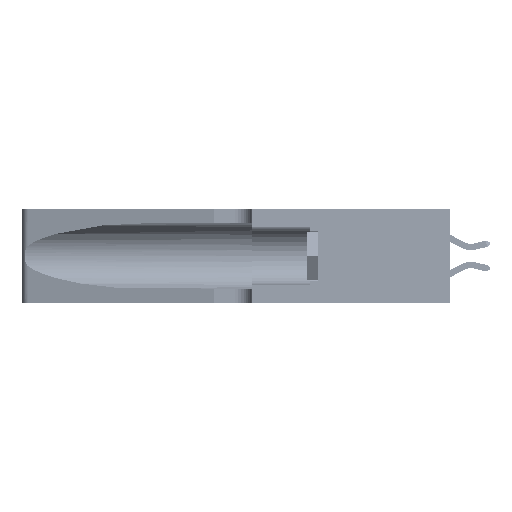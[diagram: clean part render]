
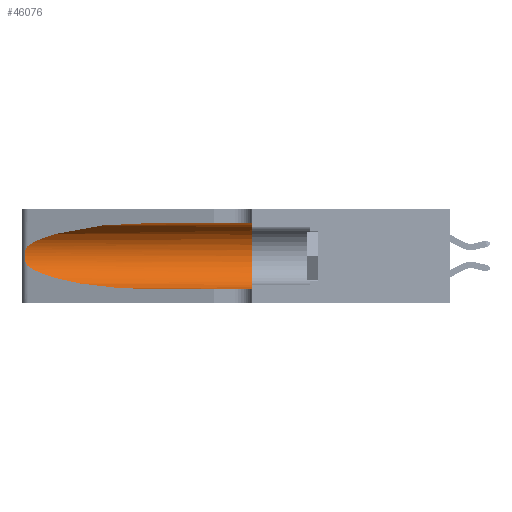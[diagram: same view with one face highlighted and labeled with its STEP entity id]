
A CAD part, left-side view. The second image highlights one B-rep face of the part: STEP entity #46076.
In plain terms, the highlighted cylindrical face has radius 3.308 mm (diameter 6.617 mm), a partial arc.
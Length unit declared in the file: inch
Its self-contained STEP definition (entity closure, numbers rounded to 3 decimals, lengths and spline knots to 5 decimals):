
#816 = DIRECTION ( 'NONE',  ( 0., 0., 1. ) ) ;
#819 = ORIENTED_EDGE ( 'NONE', *, *, #31638, .T. ) ;
#899 = CARTESIAN_POINT ( 'NONE',  ( 0.26075, 1.23896, 0.178 ) ) ;
#1541 = VERTEX_POINT ( 'NONE', #27098 ) ;
#3006 = FACE_OUTER_BOUND ( 'NONE', #21736, .T. ) ;
#5270 = CARTESIAN_POINT ( 'NONE',  ( 0.25856, 1.23593, 0.16098 ) ) ;
#9612 = CARTESIAN_POINT ( 'NONE',  ( 0.25639, 1.23186, 0.15144 ) ) ;
#9750 = AXIS2_PLACEMENT_3D ( 'NONE', #45708, #20847, #29178 ) ;
#10561 = CARTESIAN_POINT ( 'NONE',  ( 0.18966, 0.96281, 0.31525 ) ) ;
#13496 = ORIENTED_EDGE ( 'NONE', *, *, #45112, .T. ) ;
#13919 = CARTESIAN_POINT ( 'NONE',  ( 0.25487, 1.22718, 0.14631 ) ) ;
#15225 = CARTESIAN_POINT ( 'NONE',  ( 0.25487, 1.22718, 0.14631 ) ) ;
#15286 = CARTESIAN_POINT ( 'NONE',  ( 0.1305, 0.72297, 0.31525 ) ) ;
#15536 = ORIENTED_EDGE ( 'NONE', *, *, #39988, .F. ) ;
#18020 = CARTESIAN_POINT ( 'NONE',  ( 0.25639, 1.23184, 0.21858 ) ) ;
#19123 = CARTESIAN_POINT ( 'NONE',  ( 0.1305, 0.72297, 0.31525 ) ) ;
#19491 = CARTESIAN_POINT ( 'NONE',  ( 0.2373, 1.15595, 0.08982 ) ) ;
#20099 =( BOUNDED_CURVE ( )  B_SPLINE_CURVE ( 3, ( #19123, #10561, #39635, #48132 ),
 .UNSPECIFIED., .F., .F. ) 
 B_SPLINE_CURVE_WITH_KNOTS ( ( 4, 4 ),
 ( 1.5708, 2.84003 ),
 .UNSPECIFIED. ) 
 CURVE ( )  GEOMETRIC_REPRESENTATION_ITEM ( )  RATIONAL_B_SPLINE_CURVE ( ( 1., 0.87, 0.87, 1. ) ) 
 REPRESENTATION_ITEM ( '' )  );
#20847 = DIRECTION ( 'NONE',  ( 0., -1., 0. ) ) ;
#20879 = CARTESIAN_POINT ( 'NONE',  ( 0.25487, 1.22718, 0.22369 ) ) ;
#21736 = EDGE_LOOP ( 'NONE', ( #52640, #13496, #819, #24892, #15536, #44374 ) ) ;
#22223 = CARTESIAN_POINT ( 'NONE',  ( 0.25854, 1.2359, 0.20912 ) ) ;
#23657 = CARTESIAN_POINT ( 'NONE',  ( 0.1305, 0.72297, 0.05475 ) ) ;
#24892 = ORIENTED_EDGE ( 'NONE', *, *, #35513, .T. ) ;
#25567 = EDGE_CURVE ( 'NONE', #27614, #38202, #27658, .T. ) ;
#25776 = VERTEX_POINT ( 'NONE', #36055 ) ;
#25979 = CIRCLE ( 'NONE', #46325, 0.13025 ) ;
#26283 = DIRECTION ( 'NONE',  ( 0., 1., 0. ) ) ;
#26363 = VECTOR ( 'NONE', #39151, 39.37008 ) ;
#26373 = CARTESIAN_POINT ( 'NONE',  ( 0.26075, 1.23896, 0.19203 ) ) ;
#26374 = EDGE_CURVE ( 'NONE', #27614, #29421, #20099, .T. ) ;
#27098 = CARTESIAN_POINT ( 'NONE',  ( 0.1305, 0.72297, 0.05475 ) ) ;
#27614 = VERTEX_POINT ( 'NONE', #15286 ) ;
#27658 = LINE ( 'NONE', #34994, #26363 ) ;
#28238 = VECTOR ( 'NONE', #52768, 39.37008 ) ;
#29178 = DIRECTION ( 'NONE',  ( 0., 0., -1. ) ) ;
#29421 = VERTEX_POINT ( 'NONE', #20879 ) ;
#29703 =( BOUNDED_CURVE ( )  B_SPLINE_CURVE ( 3, ( #15225, #19491, #48494, #23657 ),
 .UNSPECIFIED., .F., .F. ) 
 B_SPLINE_CURVE_WITH_KNOTS ( ( 4, 4 ),
 ( 3.44316, 4.71239 ),
 .UNSPECIFIED. ) 
 CURVE ( )  GEOMETRIC_REPRESENTATION_ITEM ( )  RATIONAL_B_SPLINE_CURVE ( ( 1., 0.87, 0.87, 1. ) ) 
 REPRESENTATION_ITEM ( '' )  );
#30538 = CARTESIAN_POINT ( 'NONE',  ( 0.26017, 1.23833, 0.17102 ) ) ;
#31638 = EDGE_CURVE ( 'NONE', #25776, #1541, #29703, .T. ) ;
#32169 = CARTESIAN_POINT ( 'NONE',  ( 0.1305, 1.61858, 0.05475 ) ) ;
#34734 = CARTESIAN_POINT ( 'NONE',  ( 0.25789, 1.23486, 0.15765 ) ) ;
#34994 = CARTESIAN_POINT ( 'NONE',  ( 0.1305, 1.61858, 0.31525 ) ) ;
#35513 = EDGE_CURVE ( 'NONE', #1541, #40573, #39302, .T. ) ;
#36055 = CARTESIAN_POINT ( 'NONE',  ( 0.25487, 1.22718, 0.14631 ) ) ;
#38202 = VERTEX_POINT ( 'NONE', #48040 ) ;
#38731 = CARTESIAN_POINT ( 'NONE',  ( 0.25487, 1.22718, 0.22369 ) ) ;
#38899 = CARTESIAN_POINT ( 'NONE',  ( 0.25555, 1.22993, 0.14849 ) ) ;
#39151 = DIRECTION ( 'NONE',  ( 0., -1., 0. ) ) ;
#39302 = LINE ( 'NONE', #32169, #28238 ) ;
#39635 = CARTESIAN_POINT ( 'NONE',  ( 0.2373, 1.15595, 0.28018 ) ) ;
#39988 = EDGE_CURVE ( 'NONE', #38202, #40573, #25979, .T. ) ;
#40573 = VERTEX_POINT ( 'NONE', #42472 ) ;
#42472 = CARTESIAN_POINT ( 'NONE',  ( 0.1305, 0.35, 0.05475 ) ) ;
#42891 = CARTESIAN_POINT ( 'NONE',  ( 0.25555, 1.22994, 0.2215 ) ) ;
#43384 = B_SPLINE_CURVE_WITH_KNOTS ( 'NONE', 3,
 ( #38731, #42891, #18020, #47047, #22223, #51205, #26373, #899, #30538, #5270, #34734, #9612, #38899, #13919 ),
 .UNSPECIFIED., .F., .F.,
 ( 4, 2, 2, 2, 2, 2, 4 ),
 ( 0., 0.00027, 0.00053, 0.00107, 0.0016, 0.00187, 0.00214 ),
 .UNSPECIFIED. ) ;
#43772 = CYLINDRICAL_SURFACE ( 'NONE', #9750, 0.13025 ) ;
#44374 = ORIENTED_EDGE ( 'NONE', *, *, #25567, .F. ) ;
#45112 = EDGE_CURVE ( 'NONE', #29421, #25776, #43384, .T. ) ;
#45708 = CARTESIAN_POINT ( 'NONE',  ( 0.1305, 1.61858, 0.185 ) ) ;
#46076 = ADVANCED_FACE ( 'NONE', ( #3006 ), #43772, .F. ) ;
#46325 = AXIS2_PLACEMENT_3D ( 'NONE', #51125, #26283, #816 ) ;
#47047 = CARTESIAN_POINT ( 'NONE',  ( 0.25787, 1.23484, 0.2124 ) ) ;
#48040 = CARTESIAN_POINT ( 'NONE',  ( 0.1305, 0.35, 0.31525 ) ) ;
#48132 = CARTESIAN_POINT ( 'NONE',  ( 0.25487, 1.22718, 0.22369 ) ) ;
#48494 = CARTESIAN_POINT ( 'NONE',  ( 0.18966, 0.96281, 0.05475 ) ) ;
#51125 = CARTESIAN_POINT ( 'NONE',  ( 0.1305, 0.35, 0.185 ) ) ;
#51205 = CARTESIAN_POINT ( 'NONE',  ( 0.26018, 1.23835, 0.19895 ) ) ;
#52640 = ORIENTED_EDGE ( 'NONE', *, *, #26374, .T. ) ;
#52768 = DIRECTION ( 'NONE',  ( 0., -1., 0. ) ) ;
